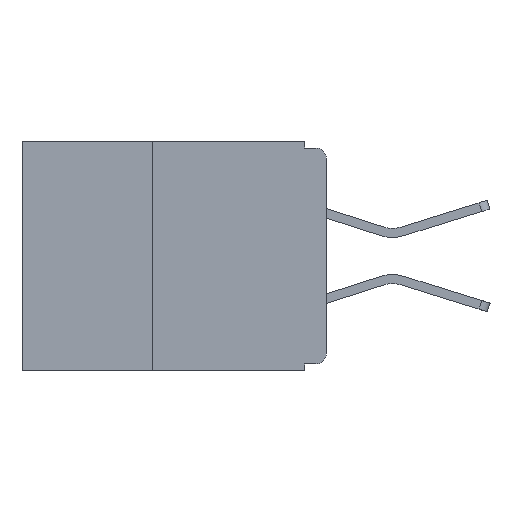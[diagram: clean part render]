
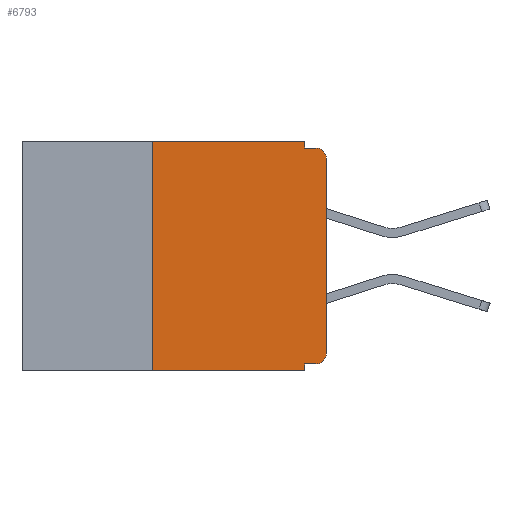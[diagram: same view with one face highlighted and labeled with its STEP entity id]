
A CAD part, left-side view. The second image highlights one B-rep face of the part: STEP entity #6793.
In plain terms, the highlighted planar face has unit normal (-1, 0, 0).
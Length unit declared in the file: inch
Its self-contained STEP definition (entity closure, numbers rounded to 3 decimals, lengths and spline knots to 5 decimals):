
#188 = CARTESIAN_POINT ( 'NONE',  ( 0., 0., -0.32 ) ) ;
#287 = LINE ( 'NONE', #10279, #2109 ) ;
#397 = VECTOR ( 'NONE', #9185, 39.37008 ) ;
#465 = ORIENTED_EDGE ( 'NONE', *, *, #2941, .F. ) ;
#468 = DIRECTION ( 'NONE',  ( 0., 0., -1. ) ) ;
#583 = EDGE_CURVE ( 'NONE', #6694, #3926, #11157, .T. ) ;
#827 = CIRCLE ( 'NONE', #5292, 0.015 ) ;
#1744 = EDGE_LOOP ( 'NONE', ( #2953, #10768, #9478, #5993, #8401, #11665, #3184, #465, #10433, #7426 ) ) ;
#1831 = DIRECTION ( 'NONE',  ( 0., 0., -1. ) ) ;
#1963 = CARTESIAN_POINT ( 'NONE',  ( 0., 0.031, -0.32 ) ) ;
#2109 = VECTOR ( 'NONE', #11160, 39.37008 ) ;
#2416 = EDGE_CURVE ( 'NONE', #5684, #11482, #9488, .T. ) ;
#2698 = EDGE_CURVE ( 'NONE', #10517, #9306, #6011, .T. ) ;
#2736 = EDGE_CURVE ( 'NONE', #11482, #5709, #8198, .T. ) ;
#2748 = DIRECTION ( 'NONE',  ( -1., 0., 0. ) ) ;
#2762 = CARTESIAN_POINT ( 'NONE',  ( 0., 0.015, -0.305 ) ) ;
#2941 = EDGE_CURVE ( 'NONE', #4779, #7174, #3848, .T. ) ;
#2953 = ORIENTED_EDGE ( 'NONE', *, *, #2736, .T. ) ;
#2983 = VECTOR ( 'NONE', #8000, 39.37008 ) ;
#3184 = ORIENTED_EDGE ( 'NONE', *, *, #8064, .T. ) ;
#3407 = VECTOR ( 'NONE', #10396, 39.37008 ) ;
#3465 = AXIS2_PLACEMENT_3D ( 'NONE', #2762, #2748, #468 ) ;
#3848 = LINE ( 'NONE', #5518, #8906 ) ;
#3926 = VERTEX_POINT ( 'NONE', #7849 ) ;
#4423 = EDGE_CURVE ( 'NONE', #5709, #6040, #827, .T. ) ;
#4507 = LINE ( 'NONE', #8625, #11595 ) ;
#4607 = CARTESIAN_POINT ( 'NONE',  ( 0., 0.015, -0.01 ) ) ;
#4635 = DIRECTION ( 'NONE',  ( 0., 0., -1. ) ) ;
#4667 = DIRECTION ( 'NONE',  ( -1., 0., 0. ) ) ;
#4672 = CARTESIAN_POINT ( 'NONE',  ( 0., 0.015, -0.025 ) ) ;
#4779 = VERTEX_POINT ( 'NONE', #1963 ) ;
#5138 = CARTESIAN_POINT ( 'NONE',  ( 0., 0.437, 0. ) ) ;
#5292 = AXIS2_PLACEMENT_3D ( 'NONE', #4672, #4667, #4635 ) ;
#5300 = CARTESIAN_POINT ( 'NONE',  ( 0., 0.031, 0. ) ) ;
#5430 = DIRECTION ( 'NONE',  ( 0., 0., -1. ) ) ;
#5518 = CARTESIAN_POINT ( 'NONE',  ( 0., 0.031, -0.33 ) ) ;
#5532 = CARTESIAN_POINT ( 'NONE',  ( 0., 0.031, -0.01 ) ) ;
#5579 = CARTESIAN_POINT ( 'NONE',  ( 0., 0.25, -0.33 ) ) ;
#5684 = VERTEX_POINT ( 'NONE', #9770 ) ;
#5709 = VERTEX_POINT ( 'NONE', #9810 ) ;
#5862 = LINE ( 'NONE', #5138, #2983 ) ;
#5993 = ORIENTED_EDGE ( 'NONE', *, *, #2698, .F. ) ;
#6011 = LINE ( 'NONE', #10089, #3407 ) ;
#6040 = VERTEX_POINT ( 'NONE', #4607 ) ;
#6203 = CARTESIAN_POINT ( 'NONE',  ( 0., 0., -0.305 ) ) ;
#6694 = VERTEX_POINT ( 'NONE', #5579 ) ;
#6793 = ADVANCED_FACE ( 'NONE', ( #10211 ), #11171, .F. ) ;
#6898 = LINE ( 'NONE', #188, #9030 ) ;
#7174 = VERTEX_POINT ( 'NONE', #10803 ) ;
#7260 = EDGE_CURVE ( 'NONE', #9306, #6040, #287, .T. ) ;
#7426 = ORIENTED_EDGE ( 'NONE', *, *, #2416, .T. ) ;
#7615 = DIRECTION ( 'NONE',  ( 1., 0., 0. ) ) ;
#7849 = CARTESIAN_POINT ( 'NONE',  ( 0., 0.25, 0. ) ) ;
#8000 = DIRECTION ( 'NONE',  ( 0., -1., 0. ) ) ;
#8043 = DIRECTION ( 'NONE',  ( 0., 1., 0. ) ) ;
#8064 = EDGE_CURVE ( 'NONE', #6694, #7174, #4507, .T. ) ;
#8198 = LINE ( 'NONE', #9503, #397 ) ;
#8202 = CARTESIAN_POINT ( 'NONE',  ( 0., 0.25, -0.33 ) ) ;
#8401 = ORIENTED_EDGE ( 'NONE', *, *, #10438, .F. ) ;
#8625 = CARTESIAN_POINT ( 'NONE',  ( 0., 0.437, -0.33 ) ) ;
#8906 = VECTOR ( 'NONE', #5430, 39.37008 ) ;
#9030 = VECTOR ( 'NONE', #8043, 39.37008 ) ;
#9185 = DIRECTION ( 'NONE',  ( 0., 0., 1. ) ) ;
#9217 = AXIS2_PLACEMENT_3D ( 'NONE', #11124, #7615, #1831 ) ;
#9306 = VERTEX_POINT ( 'NONE', #5532 ) ;
#9478 = ORIENTED_EDGE ( 'NONE', *, *, #7260, .F. ) ;
#9488 = CIRCLE ( 'NONE', #3465, 0.015 ) ;
#9503 = CARTESIAN_POINT ( 'NONE',  ( 0., 0., 0. ) ) ;
#9646 = DIRECTION ( 'NONE',  ( 0., 0., 1. ) ) ;
#9770 = CARTESIAN_POINT ( 'NONE',  ( 0., 0.015, -0.32 ) ) ;
#9810 = CARTESIAN_POINT ( 'NONE',  ( 0., 0., -0.025 ) ) ;
#10089 = CARTESIAN_POINT ( 'NONE',  ( 0., 0.031, 0. ) ) ;
#10211 = FACE_OUTER_BOUND ( 'NONE', #1744, .T. ) ;
#10279 = CARTESIAN_POINT ( 'NONE',  ( 0., 0., -0.01 ) ) ;
#10396 = DIRECTION ( 'NONE',  ( 0., 0., -1. ) ) ;
#10433 = ORIENTED_EDGE ( 'NONE', *, *, #11467, .F. ) ;
#10438 = EDGE_CURVE ( 'NONE', #3926, #10517, #5862, .T. ) ;
#10517 = VERTEX_POINT ( 'NONE', #5300 ) ;
#10768 = ORIENTED_EDGE ( 'NONE', *, *, #4423, .T. ) ;
#10803 = CARTESIAN_POINT ( 'NONE',  ( 0., 0.031, -0.33 ) ) ;
#10867 = VECTOR ( 'NONE', #9646, 39.37008 ) ;
#11124 = CARTESIAN_POINT ( 'NONE',  ( 0., 0.437, 0. ) ) ;
#11157 = LINE ( 'NONE', #8202, #10867 ) ;
#11160 = DIRECTION ( 'NONE',  ( 0., -1., 0. ) ) ;
#11171 = PLANE ( 'NONE',  #9217 ) ;
#11467 = EDGE_CURVE ( 'NONE', #5684, #4779, #6898, .T. ) ;
#11482 = VERTEX_POINT ( 'NONE', #6203 ) ;
#11595 = VECTOR ( 'NONE', #12129, 39.37008 ) ;
#11665 = ORIENTED_EDGE ( 'NONE', *, *, #583, .F. ) ;
#12129 = DIRECTION ( 'NONE',  ( 0., -1., 0. ) ) ;
